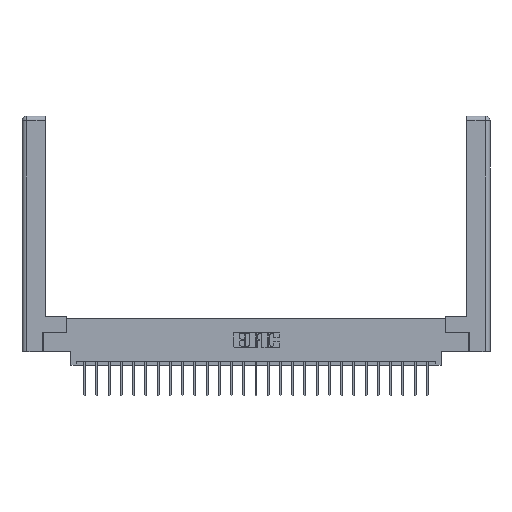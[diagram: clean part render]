
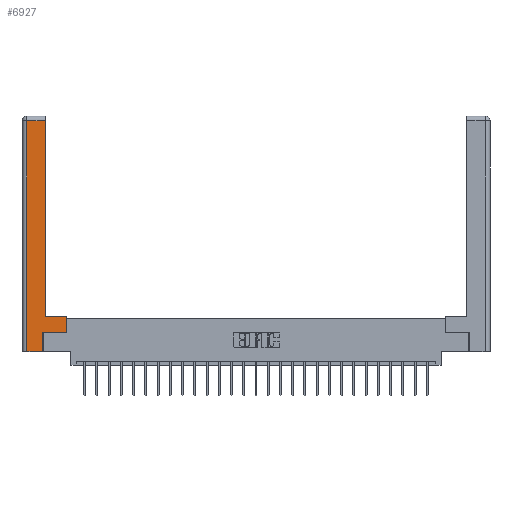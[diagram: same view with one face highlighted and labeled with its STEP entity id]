
A CAD part, top view. The second image highlights one B-rep face of the part: STEP entity #6927.
In plain terms, the highlighted planar face has unit normal (0, 0, 1).
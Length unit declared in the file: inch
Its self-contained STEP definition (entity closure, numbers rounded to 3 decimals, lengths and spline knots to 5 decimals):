
#16 = VECTOR ( 'NONE', #16806, 39.37008 ) ;
#450 = DIRECTION ( 'NONE',  ( -1., 0., 0. ) ) ;
#711 = LINE ( 'NONE', #24413, #22163 ) ;
#764 = ORIENTED_EDGE ( 'NONE', *, *, #5678, .T. ) ;
#1982 = CARTESIAN_POINT ( 'NONE',  ( 0.265, 0.245, 0. ) ) ;
#2663 = LINE ( 'NONE', #25394, #15344 ) ;
#3332 = LINE ( 'NONE', #8064, #16 ) ;
#3454 = VERTEX_POINT ( 'NONE', #16885 ) ;
#3547 = EDGE_CURVE ( 'NONE', #3454, #18127, #25647, .T. ) ;
#4137 = VERTEX_POINT ( 'NONE', #15826 ) ;
#4439 = VECTOR ( 'NONE', #24745, 39.37008 ) ;
#4885 = ORIENTED_EDGE ( 'NONE', *, *, #26693, .T. ) ;
#5377 = ORIENTED_EDGE ( 'NONE', *, *, #7051, .T. ) ;
#5633 = DIRECTION ( 'NONE',  ( 0., 1., 0. ) ) ;
#5678 = EDGE_CURVE ( 'NONE', #12528, #3454, #25859, .T. ) ;
#6558 = EDGE_CURVE ( 'NONE', #9221, #4137, #17628, .T. ) ;
#6598 = EDGE_CURVE ( 'NONE', #20513, #9174, #711, .T. ) ;
#6927 = ADVANCED_FACE ( 'NONE', ( #12142 ), #16826, .F. ) ;
#7051 = EDGE_CURVE ( 'NONE', #9174, #12528, #2663, .T. ) ;
#7685 = VECTOR ( 'NONE', #23714, 39.37008 ) ;
#7852 = DIRECTION ( 'NONE',  ( 1., 0., 0. ) ) ;
#8064 = CARTESIAN_POINT ( 'NONE',  ( 0.565, 0.45, 0. ) ) ;
#8075 = DIRECTION ( 'NONE',  ( 0., 0., -1. ) ) ;
#8175 = CARTESIAN_POINT ( 'NONE',  ( 0.295, 0.45, 0. ) ) ;
#8527 = DIRECTION ( 'NONE',  ( -1., 0., 0. ) ) ;
#9174 = VERTEX_POINT ( 'NONE', #23217 ) ;
#9221 = VERTEX_POINT ( 'NONE', #25817 ) ;
#10214 = AXIS2_PLACEMENT_3D ( 'NONE', #10712, #8075, #8527 ) ;
#10712 = CARTESIAN_POINT ( 'NONE',  ( 0., 0., 0. ) ) ;
#11816 = EDGE_CURVE ( 'NONE', #18127, #9221, #14788, .T. ) ;
#12112 = CARTESIAN_POINT ( 'NONE',  ( 0.265, 0., 0. ) ) ;
#12142 = FACE_OUTER_BOUND ( 'NONE', #20394, .T. ) ;
#12528 = VERTEX_POINT ( 'NONE', #15835 ) ;
#13369 = DIRECTION ( 'NONE',  ( 1., 0., 0. ) ) ;
#14226 = VERTEX_POINT ( 'NONE', #23142 ) ;
#14788 = LINE ( 'NONE', #1982, #19935 ) ;
#15344 = VECTOR ( 'NONE', #450, 39.37008 ) ;
#15384 = CARTESIAN_POINT ( 'NONE',  ( 0.0615, 0., 0. ) ) ;
#15826 = CARTESIAN_POINT ( 'NONE',  ( 0.565, 0.245, 0. ) ) ;
#15835 = CARTESIAN_POINT ( 'NONE',  ( 0.0615, 2.94, 0. ) ) ;
#16806 = DIRECTION ( 'NONE',  ( 0., 1., 0. ) ) ;
#16826 = PLANE ( 'NONE',  #10214 ) ;
#16885 = CARTESIAN_POINT ( 'NONE',  ( 0.0615, 0., 0. ) ) ;
#17129 = ORIENTED_EDGE ( 'NONE', *, *, #19839, .T. ) ;
#17197 = ORIENTED_EDGE ( 'NONE', *, *, #6598, .T. ) ;
#17599 = CARTESIAN_POINT ( 'NONE',  ( 0.295, 0.45, 0. ) ) ;
#17628 = LINE ( 'NONE', #17870, #25122 ) ;
#17870 = CARTESIAN_POINT ( 'NONE',  ( 0.565, 0.245, 0. ) ) ;
#18127 = VERTEX_POINT ( 'NONE', #12112 ) ;
#19839 = EDGE_CURVE ( 'NONE', #4137, #14226, #3332, .T. ) ;
#19863 = ORIENTED_EDGE ( 'NONE', *, *, #3547, .T. ) ;
#19935 = VECTOR ( 'NONE', #26816, 39.37008 ) ;
#20083 = VECTOR ( 'NONE', #13369, 39.37008 ) ;
#20347 = LINE ( 'NONE', #8175, #4439 ) ;
#20394 = EDGE_LOOP ( 'NONE', ( #17197, #5377, #764, #19863, #25370, #21756, #17129, #4885 ) ) ;
#20513 = VERTEX_POINT ( 'NONE', #17599 ) ;
#21756 = ORIENTED_EDGE ( 'NONE', *, *, #6558, .T. ) ;
#22163 = VECTOR ( 'NONE', #5633, 39.37008 ) ;
#23142 = CARTESIAN_POINT ( 'NONE',  ( 0.565, 0.45, 0. ) ) ;
#23217 = CARTESIAN_POINT ( 'NONE',  ( 0.295, 2.94, 0. ) ) ;
#23714 = DIRECTION ( 'NONE',  ( 0., -1., 0. ) ) ;
#24413 = CARTESIAN_POINT ( 'NONE',  ( 0.295, 3., 0. ) ) ;
#24745 = DIRECTION ( 'NONE',  ( -1., 0., 0. ) ) ;
#25122 = VECTOR ( 'NONE', #7852, 39.37008 ) ;
#25370 = ORIENTED_EDGE ( 'NONE', *, *, #11816, .T. ) ;
#25394 = CARTESIAN_POINT ( 'NONE',  ( 0.0615, 2.94, 0. ) ) ;
#25647 = LINE ( 'NONE', #25819, #20083 ) ;
#25817 = CARTESIAN_POINT ( 'NONE',  ( 0.265, 0.245, 0. ) ) ;
#25819 = CARTESIAN_POINT ( 'NONE',  ( 0.265, 0., 0. ) ) ;
#25859 = LINE ( 'NONE', #15384, #7685 ) ;
#26693 = EDGE_CURVE ( 'NONE', #14226, #20513, #20347, .T. ) ;
#26816 = DIRECTION ( 'NONE',  ( 0., 1., 0. ) ) ;
